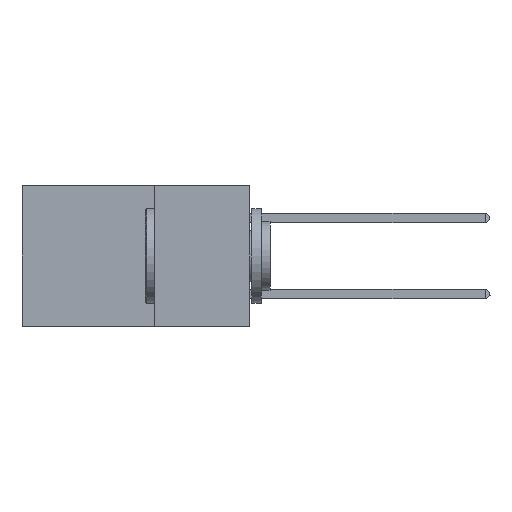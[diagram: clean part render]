
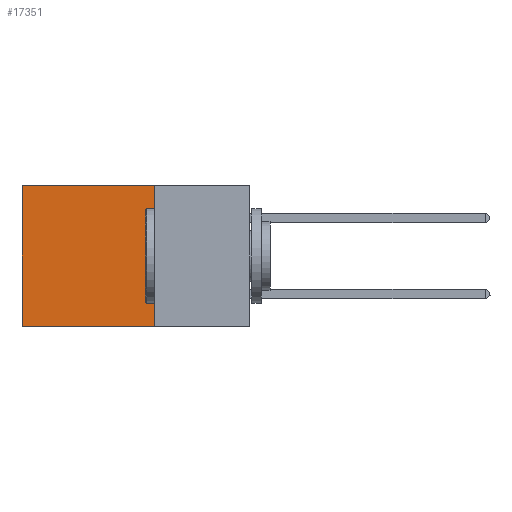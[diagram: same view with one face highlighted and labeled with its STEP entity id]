
A CAD part, left-side view. The second image highlights one B-rep face of the part: STEP entity #17351.
In plain terms, the highlighted planar face has unit normal (-1, 0, 0).
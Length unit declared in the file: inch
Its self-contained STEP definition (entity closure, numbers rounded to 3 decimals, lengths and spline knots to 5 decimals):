
#790 = CARTESIAN_POINT ( 'NONE',  ( 0.2875, 0.25, 0. ) ) ;
#874 = DIRECTION ( 'NONE',  ( 1., 0., 0. ) ) ;
#1076 = DIRECTION ( 'NONE',  ( 0., 0., -1. ) ) ;
#1926 = CARTESIAN_POINT ( 'NONE',  ( 0.2875, 0.25, -0.37 ) ) ;
#2309 = VERTEX_POINT ( 'NONE', #19809 ) ;
#3612 = EDGE_CURVE ( 'NONE', #6778, #13885, #8468, .T. ) ;
#4405 = DIRECTION ( 'NONE',  ( 0., 0., -1. ) ) ;
#4836 = LINE ( 'NONE', #790, #13601 ) ;
#5221 = CARTESIAN_POINT ( 'NONE',  ( 0.2875, 0.25, 0. ) ) ;
#6007 = LINE ( 'NONE', #1926, #25932 ) ;
#6290 = EDGE_CURVE ( 'NONE', #13885, #2309, #6652, .T. ) ;
#6652 = LINE ( 'NONE', #17213, #15435 ) ;
#6778 = VERTEX_POINT ( 'NONE', #21642 ) ;
#7339 = ORIENTED_EDGE ( 'NONE', *, *, #6290, .T. ) ;
#7381 = DIRECTION ( 'NONE',  ( 0., 1., 0. ) ) ;
#8468 = LINE ( 'NONE', #5221, #11625 ) ;
#8903 = CARTESIAN_POINT ( 'NONE',  ( 0.2875, 0.6, 0. ) ) ;
#9240 = CARTESIAN_POINT ( 'NONE',  ( 0.2875, 0.25, -0.37 ) ) ;
#11625 = VECTOR ( 'NONE', #7381, 39.37008 ) ;
#11930 = CARTESIAN_POINT ( 'NONE',  ( 0.2875, 0.25, 0. ) ) ;
#13446 = ORIENTED_EDGE ( 'NONE', *, *, #25505, .F. ) ;
#13601 = VECTOR ( 'NONE', #24343, 39.37008 ) ;
#13885 = VERTEX_POINT ( 'NONE', #8903 ) ;
#14026 = PLANE ( 'NONE',  #15701 ) ;
#14648 = FACE_OUTER_BOUND ( 'NONE', #20467, .T. ) ;
#15435 = VECTOR ( 'NONE', #4405, 39.37008 ) ;
#15701 = AXIS2_PLACEMENT_3D ( 'NONE', #11930, #874, #1076 ) ;
#17128 = ORIENTED_EDGE ( 'NONE', *, *, #3612, .T. ) ;
#17213 = CARTESIAN_POINT ( 'NONE',  ( 0.2875, 0.6, 0. ) ) ;
#17351 = ADVANCED_FACE ( 'NONE', ( #14648 ), #14026, .F. ) ;
#19777 = ORIENTED_EDGE ( 'NONE', *, *, #22661, .F. ) ;
#19809 = CARTESIAN_POINT ( 'NONE',  ( 0.2875, 0.6, -0.37 ) ) ;
#20467 = EDGE_LOOP ( 'NONE', ( #7339, #19777, #13446, #17128 ) ) ;
#21642 = CARTESIAN_POINT ( 'NONE',  ( 0.2875, 0.25, 0. ) ) ;
#22661 = EDGE_CURVE ( 'NONE', #23591, #2309, #6007, .T. ) ;
#23591 = VERTEX_POINT ( 'NONE', #9240 ) ;
#24343 = DIRECTION ( 'NONE',  ( 0., 0., -1. ) ) ;
#25505 = EDGE_CURVE ( 'NONE', #6778, #23591, #4836, .T. ) ;
#25932 = VECTOR ( 'NONE', #27499, 39.37008 ) ;
#27499 = DIRECTION ( 'NONE',  ( 0., 1., 0. ) ) ;
